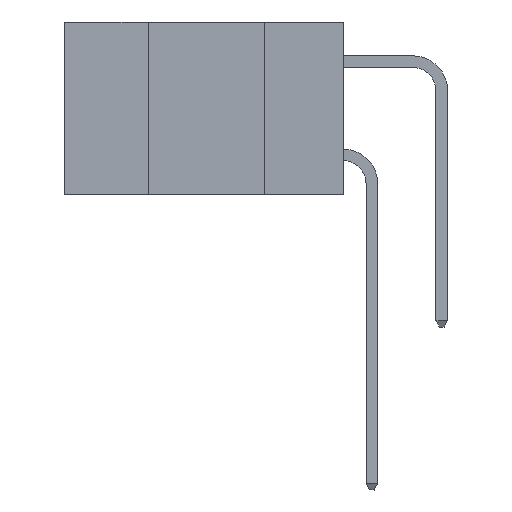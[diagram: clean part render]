
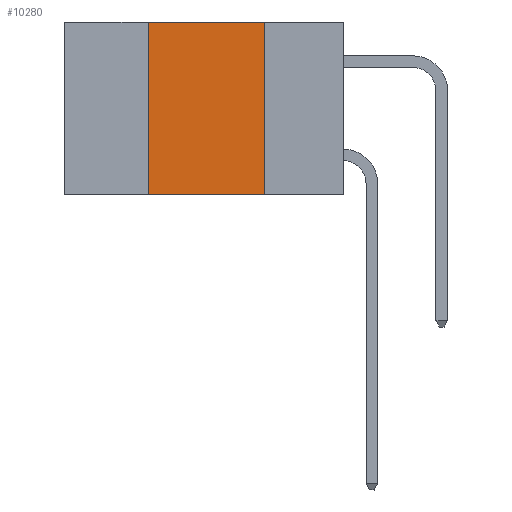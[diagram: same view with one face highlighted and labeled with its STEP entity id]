
A CAD part, left-side view. The second image highlights one B-rep face of the part: STEP entity #10280.
In plain terms, the highlighted planar face has unit normal (-1, 0, 0).
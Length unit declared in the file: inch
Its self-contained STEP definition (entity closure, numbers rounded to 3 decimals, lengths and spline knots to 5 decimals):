
#422 = EDGE_CURVE ( 'NONE', #8198, #9215, #19526, .T. ) ;
#637 = DIRECTION ( 'NONE',  ( 1., 0., 0. ) ) ;
#3465 = CARTESIAN_POINT ( 'NONE',  ( 0., 0.42, -0.37 ) ) ;
#4620 = ORIENTED_EDGE ( 'NONE', *, *, #422, .F. ) ;
#4667 = VECTOR ( 'NONE', #17888, 39.37008 ) ;
#5359 = VERTEX_POINT ( 'NONE', #19032 ) ;
#5546 = VECTOR ( 'NONE', #19402, 39.37008 ) ;
#5576 = DIRECTION ( 'NONE',  ( 0., -1., 0. ) ) ;
#5865 = DIRECTION ( 'NONE',  ( 0., 0., -1. ) ) ;
#6009 = AXIS2_PLACEMENT_3D ( 'NONE', #12579, #637, #14555 ) ;
#6035 = CARTESIAN_POINT ( 'NONE',  ( 0., 0.17, 0. ) ) ;
#8198 = VERTEX_POINT ( 'NONE', #12256 ) ;
#9215 = VERTEX_POINT ( 'NONE', #11431 ) ;
#9582 = CARTESIAN_POINT ( 'NONE',  ( 0., 0.6, -0.37 ) ) ;
#10280 = ADVANCED_FACE ( 'NONE', ( #15212 ), #18369, .F. ) ;
#11431 = CARTESIAN_POINT ( 'NONE',  ( 0., 0.17, -0.37 ) ) ;
#12106 = ORIENTED_EDGE ( 'NONE', *, *, #24567, .F. ) ;
#12256 = CARTESIAN_POINT ( 'NONE',  ( 0., 0.17, 0. ) ) ;
#12579 = CARTESIAN_POINT ( 'NONE',  ( 0., 0.6, 0. ) ) ;
#14555 = DIRECTION ( 'NONE',  ( 0., 0., -1. ) ) ;
#15212 = FACE_OUTER_BOUND ( 'NONE', #18619, .T. ) ;
#15213 = LINE ( 'NONE', #15969, #4667 ) ;
#15429 = CARTESIAN_POINT ( 'NONE',  ( 0., 0.6, 0. ) ) ;
#15969 = CARTESIAN_POINT ( 'NONE',  ( 0., 0.42, 0. ) ) ;
#17888 = DIRECTION ( 'NONE',  ( 0., 0., 1. ) ) ;
#17890 = ORIENTED_EDGE ( 'NONE', *, *, #22092, .T. ) ;
#18369 = PLANE ( 'NONE',  #6009 ) ;
#18619 = EDGE_LOOP ( 'NONE', ( #4620, #22159, #12106, #17890 ) ) ;
#19032 = CARTESIAN_POINT ( 'NONE',  ( 0., 0.42, 0. ) ) ;
#19402 = DIRECTION ( 'NONE',  ( 0., -1., 0. ) ) ;
#19526 = LINE ( 'NONE', #6035, #23454 ) ;
#20035 = VECTOR ( 'NONE', #5576, 39.37008 ) ;
#20642 = LINE ( 'NONE', #15429, #20035 ) ;
#20803 = EDGE_CURVE ( 'NONE', #5359, #8198, #20642, .T. ) ;
#21217 = LINE ( 'NONE', #9582, #5546 ) ;
#22092 = EDGE_CURVE ( 'NONE', #22687, #9215, #21217, .T. ) ;
#22159 = ORIENTED_EDGE ( 'NONE', *, *, #20803, .F. ) ;
#22687 = VERTEX_POINT ( 'NONE', #3465 ) ;
#23454 = VECTOR ( 'NONE', #5865, 39.37008 ) ;
#24567 = EDGE_CURVE ( 'NONE', #22687, #5359, #15213, .T. ) ;
